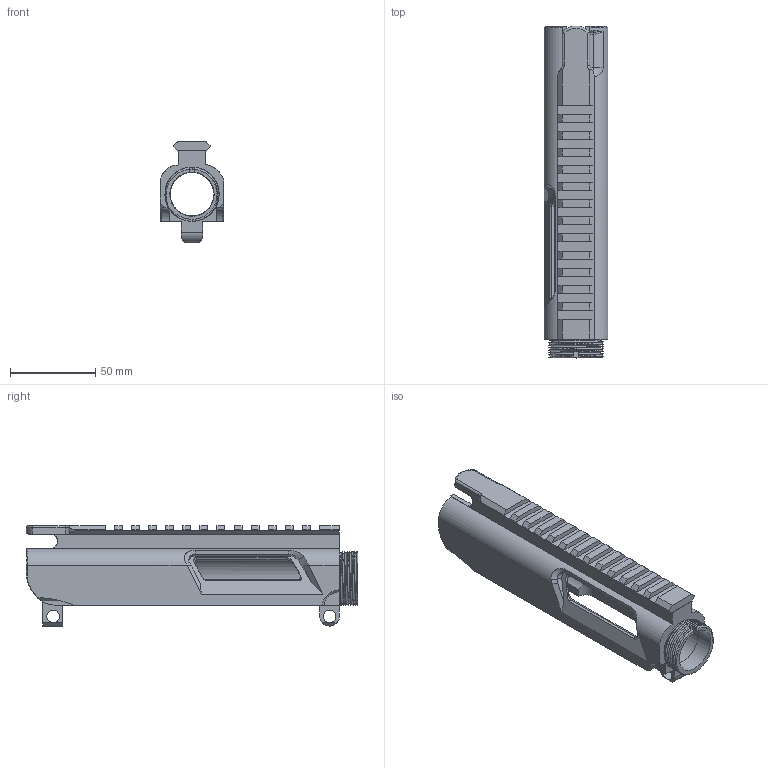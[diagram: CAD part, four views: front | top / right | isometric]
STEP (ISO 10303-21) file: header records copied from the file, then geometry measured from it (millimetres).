
FILE_DESCRIPTION(/* description */ (''),/* implementation_level */ '2;1');
FILE_NAME(/* name */ 'Slick Upper.step',/* time_stamp */ '2021-01-18T16:46:28-07:00',/* author */ (''),/* organization */ (''),/* preprocessor_version */ 'ST-DEVELOPER v18.1',/* originating_system */ 'Autodesk Translation Framework v9.7.1.1290',/* authorisation */ '');
FILE_SCHEMA (('AUTOMOTIVE_DESIGN { 1 0 10303 214 3 1 1 }'));
Length unit declared in the file: inch
Products named in the file (1): Slick Upper
Bounding box: 37.37 x 194.4 x 59 mm (x, y, z)
Volume: 111988.8 mm3; surface area: 52099 mm2
Topology: 1 solids, 1 shells, 412 faces, 1193 edges, 778 vertices
Faces by surface type: plane 240, cylinder 88, cone 50, bspline 28, torus 6
Full cylindrical faces by diameter (mm): 7.35 x1, 7.358 x1, 25.546 x1, 25.927 x1, 29.782 x1, 31.7 x4
Entity records: 16179 total; most frequent: CARTESIAN_POINT 5620, ORIENTED_EDGE 2378, DIRECTION 1952, EDGE_CURVE 1189, VERTEX_POINT 778, LINE 762, VECTOR 762, AXIS2_PLACEMENT_3D 595
